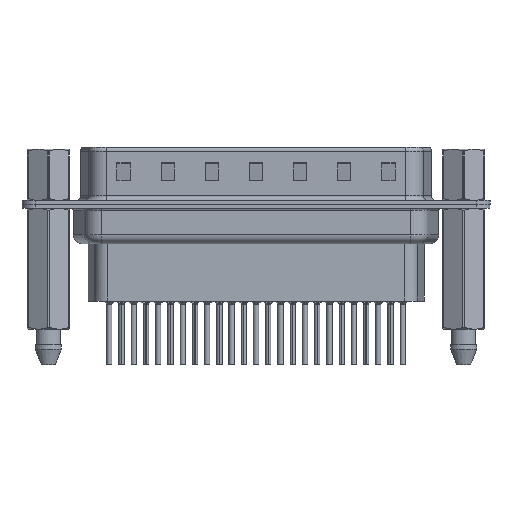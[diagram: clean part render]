
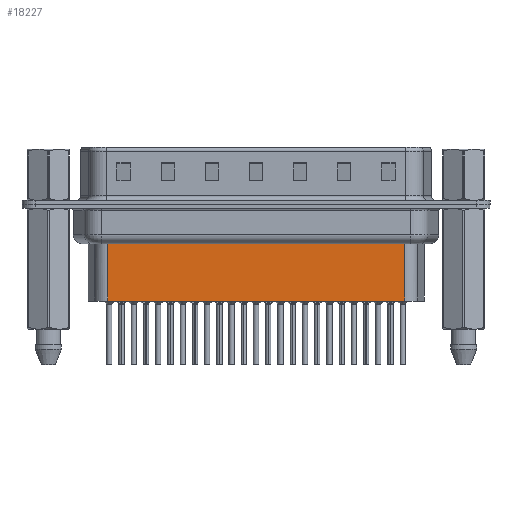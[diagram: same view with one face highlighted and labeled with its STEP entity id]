
A CAD part, front view. The second image highlights one B-rep face of the part: STEP entity #18227.
In plain terms, the highlighted planar face has unit normal (0, -1, 0).
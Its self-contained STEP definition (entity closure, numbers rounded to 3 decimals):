
#632 = FACE_OUTER_BOUND ( 'NONE', #27407, .T. ) ;
#773 = EDGE_CURVE ( 'NONE', #16886, #5599, #31694, .T. ) ;
#885 = ORIENTED_EDGE ( 'NONE', *, *, #773, .F. ) ;
#2647 = CARTESIAN_POINT ( 'NONE',  ( 6.706, -3.5, -3.1 ) ) ;
#4355 = VECTOR ( 'NONE', #31276, 1000. ) ;
#5306 = DIRECTION ( 'NONE',  ( 0., 0., -1. ) ) ;
#5599 = VERTEX_POINT ( 'NONE', #8465 ) ;
#6644 = VERTEX_POINT ( 'NONE', #18839 ) ;
#6738 = ORIENTED_EDGE ( 'NONE', *, *, #15429, .T. ) ;
#6919 = ORIENTED_EDGE ( 'NONE', *, *, #11407, .F. ) ;
#7782 = CARTESIAN_POINT ( 'NONE',  ( 6.706, -3.5, -10.95 ) ) ;
#7918 = DIRECTION ( 'NONE',  ( 0., -1., 0. ) ) ;
#8203 = LINE ( 'NONE', #18268, #4355 ) ;
#8465 = CARTESIAN_POINT ( 'NONE',  ( 6.706, -3.5, -10.95 ) ) ;
#8517 = CARTESIAN_POINT ( 'NONE',  ( 40.344, -3.5, -10.95 ) ) ;
#9213 = DIRECTION ( 'NONE',  ( 0., 0., -1. ) ) ;
#10452 = VECTOR ( 'NONE', #19979, 1000. ) ;
#11407 = EDGE_CURVE ( 'NONE', #21218, #16886, #19288, .T. ) ;
#11409 = VECTOR ( 'NONE', #5306, 1000. ) ;
#14303 = CARTESIAN_POINT ( 'NONE',  ( 40.344, -3.5, -3.1 ) ) ;
#15429 = EDGE_CURVE ( 'NONE', #21218, #6644, #8203, .T. ) ;
#16735 = ORIENTED_EDGE ( 'NONE', *, *, #21511, .T. ) ;
#16886 = VERTEX_POINT ( 'NONE', #8517 ) ;
#18227 = ADVANCED_FACE ( 'NONE', ( #632 ), #20448, .T. ) ;
#18268 = CARTESIAN_POINT ( 'NONE',  ( 6.459, -3.5, -4.097 ) ) ;
#18480 = CARTESIAN_POINT ( 'NONE',  ( 6.706, -3.5, -3.1 ) ) ;
#18839 = CARTESIAN_POINT ( 'NONE',  ( 6.706, -3.5, -4.097 ) ) ;
#19288 = LINE ( 'NONE', #14303, #27884 ) ;
#19979 = DIRECTION ( 'NONE',  ( -1., 0., 0. ) ) ;
#20448 = PLANE ( 'NONE',  #27625 ) ;
#21218 = VERTEX_POINT ( 'NONE', #22845 ) ;
#21511 = EDGE_CURVE ( 'NONE', #6644, #5599, #28405, .T. ) ;
#22845 = CARTESIAN_POINT ( 'NONE',  ( 40.344, -3.5, -4.097 ) ) ;
#27407 = EDGE_LOOP ( 'NONE', ( #6919, #6738, #16735, #885 ) ) ;
#27625 = AXIS2_PLACEMENT_3D ( 'NONE', #18480, #7918, #28378 ) ;
#27884 = VECTOR ( 'NONE', #9213, 1000. ) ;
#28378 = DIRECTION ( 'NONE',  ( 1., 0., 0. ) ) ;
#28405 = LINE ( 'NONE', #2647, #11409 ) ;
#31276 = DIRECTION ( 'NONE',  ( -1., 0., 0. ) ) ;
#31694 = LINE ( 'NONE', #7782, #10452 ) ;
